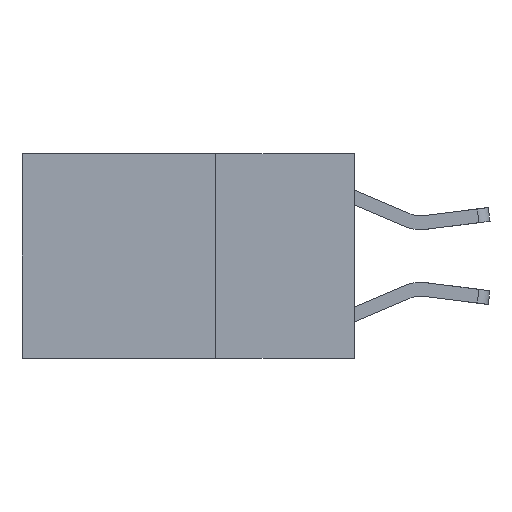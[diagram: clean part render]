
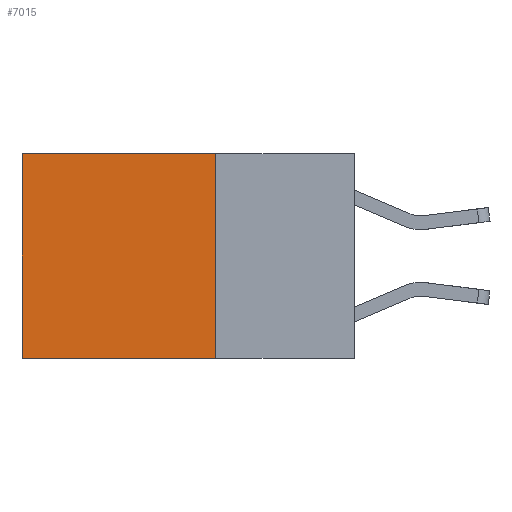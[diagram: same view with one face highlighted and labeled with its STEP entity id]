
A CAD part, left-side view. The second image highlights one B-rep face of the part: STEP entity #7015.
In plain terms, the highlighted planar face has unit normal (-1, 0, 0).
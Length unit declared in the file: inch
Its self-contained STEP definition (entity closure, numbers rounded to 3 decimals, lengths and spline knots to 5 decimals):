
#218 = CARTESIAN_POINT ( 'NONE',  ( 0.2625, 0.25, 0. ) ) ;
#301 = DIRECTION ( 'NONE',  ( 0., 0., -1. ) ) ;
#302 = DIRECTION ( 'NONE',  ( 1., 0., 0. ) ) ;
#310 = CARTESIAN_POINT ( 'NONE',  ( 0.2625, 0.25, 0. ) ) ;
#363 = PLANE ( 'NONE',  #9449 ) ;
#664 = VECTOR ( 'NONE', #7365, 39.37008 ) ;
#1024 = VECTOR ( 'NONE', #8413, 39.37008 ) ;
#1027 = VERTEX_POINT ( 'NONE', #218 ) ;
#1231 = VERTEX_POINT ( 'NONE', #7550 ) ;
#1247 = VECTOR ( 'NONE', #2748, 39.37008 ) ;
#1304 = EDGE_LOOP ( 'NONE', ( #5684, #5728, #5738, #3478 ) ) ;
#2149 = CARTESIAN_POINT ( 'NONE',  ( 0.2625, 0.25, -0.37 ) ) ;
#2206 = VECTOR ( 'NONE', #4863, 39.37008 ) ;
#2596 = CARTESIAN_POINT ( 'NONE',  ( 0.2625, 0.25, -0.37 ) ) ;
#2676 = LINE ( 'NONE', #3849, #664 ) ;
#2748 = DIRECTION ( 'NONE',  ( 0., 0., -1. ) ) ;
#3478 = ORIENTED_EDGE ( 'NONE', *, *, #9072, .T. ) ;
#3484 = EDGE_CURVE ( 'NONE', #7664, #1231, #2676, .T. ) ;
#3490 = CARTESIAN_POINT ( 'NONE',  ( 0.2625, 0.25, 0. ) ) ;
#3661 = EDGE_CURVE ( 'NONE', #1027, #6757, #5290, .T. ) ;
#3849 = CARTESIAN_POINT ( 'NONE',  ( 0.2625, 0.6, 0. ) ) ;
#4142 = CARTESIAN_POINT ( 'NONE',  ( 0.2625, 0.6, 0. ) ) ;
#4863 = DIRECTION ( 'NONE',  ( 0., 1., 0. ) ) ;
#5290 = LINE ( 'NONE', #3490, #1247 ) ;
#5623 = CARTESIAN_POINT ( 'NONE',  ( 0.2625, 0.25, 0. ) ) ;
#5684 = ORIENTED_EDGE ( 'NONE', *, *, #3484, .T. ) ;
#5728 = ORIENTED_EDGE ( 'NONE', *, *, #8417, .F. ) ;
#5738 = ORIENTED_EDGE ( 'NONE', *, *, #3661, .F. ) ;
#6510 = LINE ( 'NONE', #5623, #2206 ) ;
#6757 = VERTEX_POINT ( 'NONE', #2596 ) ;
#7015 = ADVANCED_FACE ( 'NONE', ( #9215 ), #363, .F. ) ;
#7365 = DIRECTION ( 'NONE',  ( 0., 0., -1. ) ) ;
#7550 = CARTESIAN_POINT ( 'NONE',  ( 0.2625, 0.6, -0.37 ) ) ;
#7664 = VERTEX_POINT ( 'NONE', #4142 ) ;
#8413 = DIRECTION ( 'NONE',  ( 0., 1., 0. ) ) ;
#8417 = EDGE_CURVE ( 'NONE', #6757, #1231, #9063, .T. ) ;
#9063 = LINE ( 'NONE', #2149, #1024 ) ;
#9072 = EDGE_CURVE ( 'NONE', #1027, #7664, #6510, .T. ) ;
#9215 = FACE_OUTER_BOUND ( 'NONE', #1304, .T. ) ;
#9449 = AXIS2_PLACEMENT_3D ( 'NONE', #310, #302, #301 ) ;
